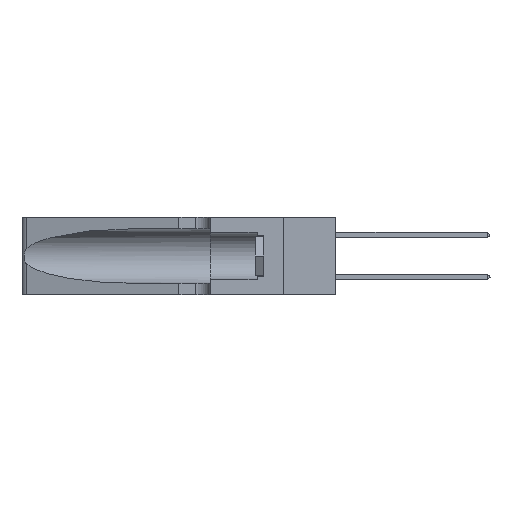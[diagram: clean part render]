
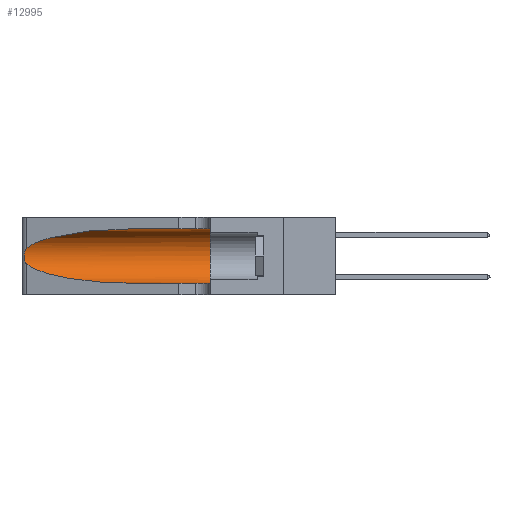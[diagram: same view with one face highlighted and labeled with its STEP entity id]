
A CAD part, left-side view. The second image highlights one B-rep face of the part: STEP entity #12995.
In plain terms, the highlighted cylindrical face has radius 3.308 mm (diameter 6.617 mm), a partial arc.
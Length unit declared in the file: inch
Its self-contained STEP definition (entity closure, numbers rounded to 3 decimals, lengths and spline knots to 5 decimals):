
#200 = DIRECTION ( 'NONE',  ( 0., 1., 0. ) ) ;
#805 = CARTESIAN_POINT ( 'NONE',  ( 0.1305, 0.35, 0.05475 ) ) ;
#2559 = CARTESIAN_POINT ( 'NONE',  ( 0.1305, 0.72297, 0.05475 ) ) ;
#2589 = CIRCLE ( 'NONE', #13603, 0.13025 ) ;
#2604 = DIRECTION ( 'NONE',  ( 0., -1., 0. ) ) ;
#3086 = CARTESIAN_POINT ( 'NONE',  ( 0.25487, 1.22718, 0.14631 ) ) ;
#3094 = CARTESIAN_POINT ( 'NONE',  ( 0.26018, 1.23835, 0.19895 ) ) ;
#3535 = EDGE_CURVE ( 'NONE', #22417, #22571, #8300, .T. ) ;
#3689 = ORIENTED_EDGE ( 'NONE', *, *, #26137, .T. ) ;
#3746 = VECTOR ( 'NONE', #2604, 39.37008 ) ;
#3975 = CARTESIAN_POINT ( 'NONE',  ( 0.1305, 1.61858, 0.31525 ) ) ;
#4491 = ORIENTED_EDGE ( 'NONE', *, *, #15397, .F. ) ;
#4647 = CARTESIAN_POINT ( 'NONE',  ( 0.1305, 0.72297, 0.31525 ) ) ;
#4830 = DIRECTION ( 'NONE',  ( 0., 0., 1. ) ) ;
#5373 = CARTESIAN_POINT ( 'NONE',  ( 0.26075, 1.23896, 0.178 ) ) ;
#5471 = CARTESIAN_POINT ( 'NONE',  ( 0.25639, 1.23186, 0.15144 ) ) ;
#6429 =( BOUNDED_CURVE ( )  B_SPLINE_CURVE ( 3, ( #29111, #26494, #28912, #29009 ),
 .UNSPECIFIED., .F., .F. ) 
 B_SPLINE_CURVE_WITH_KNOTS ( ( 4, 4 ),
 ( 1.5708, 2.84003 ),
 .UNSPECIFIED. ) 
 CURVE ( )  GEOMETRIC_REPRESENTATION_ITEM ( )  RATIONAL_B_SPLINE_CURVE ( ( 1., 0.87, 0.87, 1. ) ) 
 REPRESENTATION_ITEM ( '' )  );
#6845 = EDGE_CURVE ( 'NONE', #19751, #22417, #10609, .T. ) ;
#7561 = CARTESIAN_POINT ( 'NONE',  ( 0.25487, 1.22718, 0.14631 ) ) ;
#7872 = CARTESIAN_POINT ( 'NONE',  ( 0.25787, 1.23484, 0.2124 ) ) ;
#8300 =( BOUNDED_CURVE ( )  B_SPLINE_CURVE ( 3, ( #3086, #25343, #30042, #11961 ),
 .UNSPECIFIED., .F., .F. ) 
 B_SPLINE_CURVE_WITH_KNOTS ( ( 4, 4 ),
 ( 3.44316, 4.71239 ),
 .UNSPECIFIED. ) 
 CURVE ( )  GEOMETRIC_REPRESENTATION_ITEM ( )  RATIONAL_B_SPLINE_CURVE ( ( 1., 0.87, 0.87, 1. ) ) 
 REPRESENTATION_ITEM ( '' )  );
#9464 = VERTEX_POINT ( 'NONE', #4647 ) ;
#10570 = EDGE_LOOP ( 'NONE', ( #15515, #21485, #12672, #3689, #28021, #4491 ) ) ;
#10609 = B_SPLINE_CURVE_WITH_KNOTS ( 'NONE', 3,
 ( #26499, #24091, #21751, #7872, #22062, #3094, #21958, #5373, #27113, #27009, #19862, #5471, #22166, #7561 ),
 .UNSPECIFIED., .F., .F.,
 ( 4, 2, 2, 2, 2, 2, 4 ),
 ( 0., 0.00027, 0.00053, 0.00107, 0.0016, 0.00187, 0.00214 ),
 .UNSPECIFIED. ) ;
#10659 = CARTESIAN_POINT ( 'NONE',  ( 0.1305, 0.35, 0.31525 ) ) ;
#11129 = CARTESIAN_POINT ( 'NONE',  ( 0.1305, 1.61858, 0.185 ) ) ;
#11553 = VERTEX_POINT ( 'NONE', #805 ) ;
#11961 = CARTESIAN_POINT ( 'NONE',  ( 0.1305, 0.72297, 0.05475 ) ) ;
#12663 = CARTESIAN_POINT ( 'NONE',  ( 0.25487, 1.22718, 0.14631 ) ) ;
#12672 = ORIENTED_EDGE ( 'NONE', *, *, #3535, .T. ) ;
#12995 = ADVANCED_FACE ( 'NONE', ( #28808 ), #29539, .F. ) ;
#13603 = AXIS2_PLACEMENT_3D ( 'NONE', #16919, #200, #4830 ) ;
#13738 = DIRECTION ( 'NONE',  ( 0., -1., 0. ) ) ;
#13866 = DIRECTION ( 'NONE',  ( 0., -1., 0. ) ) ;
#14272 = LINE ( 'NONE', #16976, #3746 ) ;
#15397 = EDGE_CURVE ( 'NONE', #9464, #20211, #17155, .T. ) ;
#15515 = ORIENTED_EDGE ( 'NONE', *, *, #30966, .T. ) ;
#16919 = CARTESIAN_POINT ( 'NONE',  ( 0.1305, 0.35, 0.185 ) ) ;
#16976 = CARTESIAN_POINT ( 'NONE',  ( 0.1305, 1.61858, 0.05475 ) ) ;
#17155 = LINE ( 'NONE', #3975, #24637 ) ;
#19101 = AXIS2_PLACEMENT_3D ( 'NONE', #11129, #13866, #21097 ) ;
#19751 = VERTEX_POINT ( 'NONE', #22923 ) ;
#19862 = CARTESIAN_POINT ( 'NONE',  ( 0.25789, 1.23486, 0.15765 ) ) ;
#20211 = VERTEX_POINT ( 'NONE', #10659 ) ;
#21097 = DIRECTION ( 'NONE',  ( 0., 0., -1. ) ) ;
#21485 = ORIENTED_EDGE ( 'NONE', *, *, #6845, .T. ) ;
#21751 = CARTESIAN_POINT ( 'NONE',  ( 0.25639, 1.23184, 0.21858 ) ) ;
#21958 = CARTESIAN_POINT ( 'NONE',  ( 0.26075, 1.23896, 0.19203 ) ) ;
#22062 = CARTESIAN_POINT ( 'NONE',  ( 0.25854, 1.2359, 0.20912 ) ) ;
#22166 = CARTESIAN_POINT ( 'NONE',  ( 0.25555, 1.22993, 0.14849 ) ) ;
#22417 = VERTEX_POINT ( 'NONE', #12663 ) ;
#22571 = VERTEX_POINT ( 'NONE', #2559 ) ;
#22923 = CARTESIAN_POINT ( 'NONE',  ( 0.25487, 1.22718, 0.22369 ) ) ;
#24091 = CARTESIAN_POINT ( 'NONE',  ( 0.25555, 1.22994, 0.2215 ) ) ;
#24637 = VECTOR ( 'NONE', #13738, 39.37008 ) ;
#25343 = CARTESIAN_POINT ( 'NONE',  ( 0.2373, 1.15595, 0.08982 ) ) ;
#26137 = EDGE_CURVE ( 'NONE', #22571, #11553, #14272, .T. ) ;
#26494 = CARTESIAN_POINT ( 'NONE',  ( 0.18966, 0.96281, 0.31525 ) ) ;
#26499 = CARTESIAN_POINT ( 'NONE',  ( 0.25487, 1.22718, 0.22369 ) ) ;
#26562 = EDGE_CURVE ( 'NONE', #20211, #11553, #2589, .T. ) ;
#27009 = CARTESIAN_POINT ( 'NONE',  ( 0.25856, 1.23593, 0.16098 ) ) ;
#27113 = CARTESIAN_POINT ( 'NONE',  ( 0.26017, 1.23833, 0.17102 ) ) ;
#28021 = ORIENTED_EDGE ( 'NONE', *, *, #26562, .F. ) ;
#28808 = FACE_OUTER_BOUND ( 'NONE', #10570, .T. ) ;
#28912 = CARTESIAN_POINT ( 'NONE',  ( 0.2373, 1.15595, 0.28018 ) ) ;
#29009 = CARTESIAN_POINT ( 'NONE',  ( 0.25487, 1.22718, 0.22369 ) ) ;
#29111 = CARTESIAN_POINT ( 'NONE',  ( 0.1305, 0.72297, 0.31525 ) ) ;
#29539 = CYLINDRICAL_SURFACE ( 'NONE', #19101, 0.13025 ) ;
#30042 = CARTESIAN_POINT ( 'NONE',  ( 0.18966, 0.96281, 0.05475 ) ) ;
#30966 = EDGE_CURVE ( 'NONE', #9464, #19751, #6429, .T. ) ;
